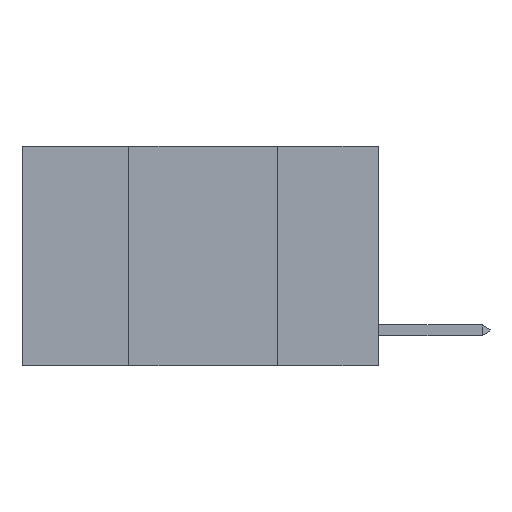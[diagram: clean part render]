
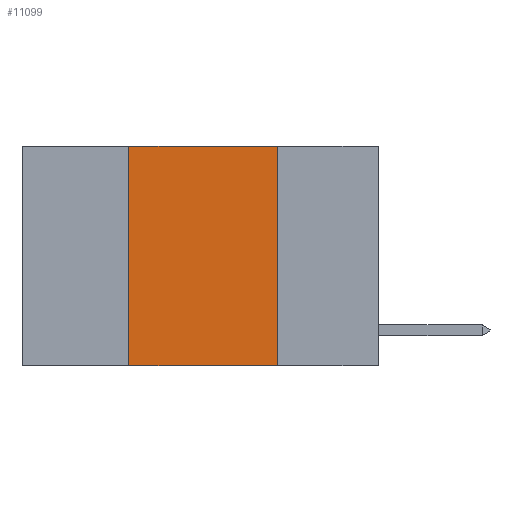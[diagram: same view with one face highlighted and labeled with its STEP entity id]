
A CAD part, left-side view. The second image highlights one B-rep face of the part: STEP entity #11099.
In plain terms, the highlighted planar face has unit normal (-1, 0, 0).
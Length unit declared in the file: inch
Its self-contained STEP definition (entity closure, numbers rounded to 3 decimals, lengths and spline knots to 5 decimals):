
#102 = VERTEX_POINT ( 'NONE', #4326 ) ;
#614 = CARTESIAN_POINT ( 'NONE',  ( 0., 0.42, 0. ) ) ;
#1419 = ORIENTED_EDGE ( 'NONE', *, *, #2141, .T. ) ;
#1539 = VECTOR ( 'NONE', #8278, 39.37008 ) ;
#1604 = VERTEX_POINT ( 'NONE', #12816 ) ;
#2141 = EDGE_CURVE ( 'NONE', #2942, #1604, #3935, .T. ) ;
#2942 = VERTEX_POINT ( 'NONE', #3533 ) ;
#3287 = VECTOR ( 'NONE', #16397, 39.37008 ) ;
#3533 = CARTESIAN_POINT ( 'NONE',  ( 0., 0.42, -0.37 ) ) ;
#3887 = VECTOR ( 'NONE', #14157, 39.37008 ) ;
#3935 = LINE ( 'NONE', #5293, #7065 ) ;
#4326 = CARTESIAN_POINT ( 'NONE',  ( 0., 0.17, 0. ) ) ;
#4353 = DIRECTION ( 'NONE',  ( 1., 0., 0. ) ) ;
#4772 = EDGE_LOOP ( 'NONE', ( #12709, #11582, #14755, #1419 ) ) ;
#5293 = CARTESIAN_POINT ( 'NONE',  ( 0., 0.6, -0.37 ) ) ;
#5655 = VERTEX_POINT ( 'NONE', #10730 ) ;
#5798 = LINE ( 'NONE', #614, #1539 ) ;
#6392 = LINE ( 'NONE', #11608, #3887 ) ;
#6908 = EDGE_CURVE ( 'NONE', #5655, #102, #12621, .T. ) ;
#7065 = VECTOR ( 'NONE', #16819, 39.37008 ) ;
#8196 = PLANE ( 'NONE',  #10983 ) ;
#8275 = FACE_OUTER_BOUND ( 'NONE', #4772, .T. ) ;
#8278 = DIRECTION ( 'NONE',  ( 0., 0., 1. ) ) ;
#10509 = EDGE_CURVE ( 'NONE', #102, #1604, #6392, .T. ) ;
#10730 = CARTESIAN_POINT ( 'NONE',  ( 0., 0.42, 0. ) ) ;
#10983 = AXIS2_PLACEMENT_3D ( 'NONE', #13471, #4353, #11842 ) ;
#11099 = ADVANCED_FACE ( 'NONE', ( #8275 ), #8196, .F. ) ;
#11582 = ORIENTED_EDGE ( 'NONE', *, *, #6908, .F. ) ;
#11608 = CARTESIAN_POINT ( 'NONE',  ( 0., 0.17, 0. ) ) ;
#11842 = DIRECTION ( 'NONE',  ( 0., 0., -1. ) ) ;
#12621 = LINE ( 'NONE', #16729, #3287 ) ;
#12709 = ORIENTED_EDGE ( 'NONE', *, *, #10509, .F. ) ;
#12816 = CARTESIAN_POINT ( 'NONE',  ( 0., 0.17, -0.37 ) ) ;
#13471 = CARTESIAN_POINT ( 'NONE',  ( 0., 0.6, 0. ) ) ;
#14157 = DIRECTION ( 'NONE',  ( 0., 0., -1. ) ) ;
#14755 = ORIENTED_EDGE ( 'NONE', *, *, #14821, .F. ) ;
#14821 = EDGE_CURVE ( 'NONE', #2942, #5655, #5798, .T. ) ;
#16397 = DIRECTION ( 'NONE',  ( 0., -1., 0. ) ) ;
#16729 = CARTESIAN_POINT ( 'NONE',  ( 0., 0.6, 0. ) ) ;
#16819 = DIRECTION ( 'NONE',  ( 0., -1., 0. ) ) ;
